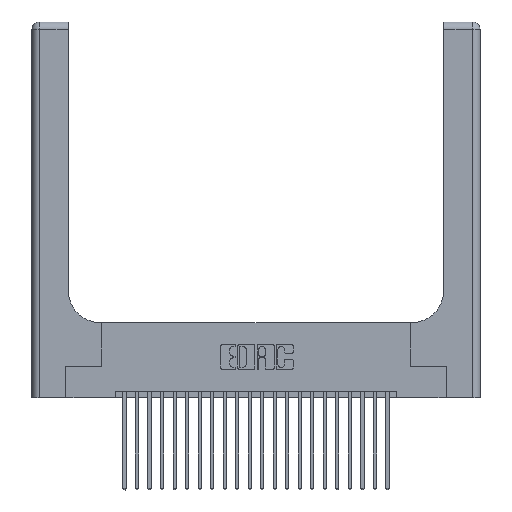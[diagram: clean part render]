
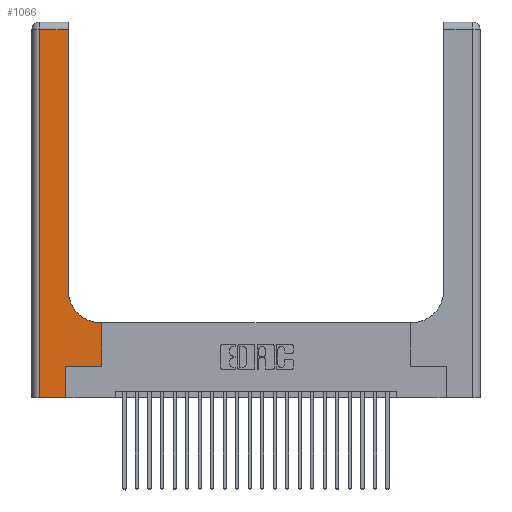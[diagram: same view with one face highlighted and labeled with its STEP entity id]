
A CAD part, top view. The second image highlights one B-rep face of the part: STEP entity #1066.
In plain terms, the highlighted planar face has unit normal (0, 0, 1).
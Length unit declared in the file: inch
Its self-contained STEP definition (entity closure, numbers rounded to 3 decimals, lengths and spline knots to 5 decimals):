
#1 = VERTEX_POINT ( 'NONE', #12243 ) ;
#51 = LINE ( 'NONE', #18129, #17416 ) ;
#165 = VERTEX_POINT ( 'NONE', #3854 ) ;
#201 = CARTESIAN_POINT ( 'NONE',  ( 0.06, 2.94, 0.37 ) ) ;
#372 = CARTESIAN_POINT ( 'NONE',  ( 0.269, 0., 0.37 ) ) ;
#1066 = ADVANCED_FACE ( 'NONE', ( #23829 ), #7288, .F. ) ;
#1139 = LINE ( 'NONE', #4367, #16083 ) ;
#1399 = ORIENTED_EDGE ( 'NONE', *, *, #13360, .T. ) ;
#2726 = DIRECTION ( 'NONE',  ( 0., 1., 0. ) ) ;
#2773 = EDGE_CURVE ( 'NONE', #1, #10433, #24336, .T. ) ;
#2787 = DIRECTION ( 'NONE',  ( 0., -1., 0. ) ) ;
#3617 = EDGE_CURVE ( 'NONE', #10433, #17808, #4555, .T. ) ;
#3854 = CARTESIAN_POINT ( 'NONE',  ( 0.2915, 2.94, 0.37 ) ) ;
#4098 = ORIENTED_EDGE ( 'NONE', *, *, #11255, .T. ) ;
#4186 = CARTESIAN_POINT ( 'NONE',  ( 0.2915, 0.6, 0.37 ) ) ;
#4367 = CARTESIAN_POINT ( 'NONE',  ( 0., 0., 0.37 ) ) ;
#4410 = CARTESIAN_POINT ( 'NONE',  ( 0.5415, 0.6, 0.37 ) ) ;
#4555 = CIRCLE ( 'NONE', #10323, 0.25 ) ;
#4596 = EDGE_CURVE ( 'NONE', #165, #16247, #18824, .T. ) ;
#5061 = ORIENTED_EDGE ( 'NONE', *, *, #21890, .T. ) ;
#5188 = CARTESIAN_POINT ( 'NONE',  ( 0.06, 0., 0.37 ) ) ;
#6261 = DIRECTION ( 'NONE',  ( 1., 0., 0. ) ) ;
#7288 = PLANE ( 'NONE',  #8512 ) ;
#7965 = CARTESIAN_POINT ( 'NONE',  ( 0., 2.94, 0.37 ) ) ;
#8123 = CARTESIAN_POINT ( 'NONE',  ( 0.269, 0.25, 0.37 ) ) ;
#8213 = EDGE_CURVE ( 'NONE', #17808, #165, #15275, .T. ) ;
#8512 = AXIS2_PLACEMENT_3D ( 'NONE', #21055, #14872, #22751 ) ;
#8567 = VECTOR ( 'NONE', #21155, 39.37008 ) ;
#8669 = DIRECTION ( 'NONE',  ( 0., 1., 0. ) ) ;
#9030 = VERTEX_POINT ( 'NONE', #372 ) ;
#10037 = VECTOR ( 'NONE', #23567, 39.37008 ) ;
#10323 = AXIS2_PLACEMENT_3D ( 'NONE', #20805, #24700, #15038 ) ;
#10433 = VERTEX_POINT ( 'NONE', #4410 ) ;
#11001 = LINE ( 'NONE', #21067, #8567 ) ;
#11255 = EDGE_CURVE ( 'NONE', #17013, #9030, #1139, .T. ) ;
#12243 = CARTESIAN_POINT ( 'NONE',  ( 0.5585, 0.6, 0.37 ) ) ;
#12869 = VERTEX_POINT ( 'NONE', #18368 ) ;
#13360 = EDGE_CURVE ( 'NONE', #16247, #17013, #19558, .T. ) ;
#14153 = DIRECTION ( 'NONE',  ( -1., 0., 0. ) ) ;
#14264 = VERTEX_POINT ( 'NONE', #19247 ) ;
#14445 = VECTOR ( 'NONE', #21695, 39.37008 ) ;
#14537 = ORIENTED_EDGE ( 'NONE', *, *, #4596, .T. ) ;
#14872 = DIRECTION ( 'NONE',  ( 0., 0., -1. ) ) ;
#15038 = DIRECTION ( 'NONE',  ( 1., 0., 0. ) ) ;
#15275 = LINE ( 'NONE', #18108, #15594 ) ;
#15594 = VECTOR ( 'NONE', #2726, 39.37008 ) ;
#16083 = VECTOR ( 'NONE', #6261, 39.37008 ) ;
#16247 = VERTEX_POINT ( 'NONE', #201 ) ;
#16311 = EDGE_CURVE ( 'NONE', #12869, #14264, #25086, .T. ) ;
#16520 = ORIENTED_EDGE ( 'NONE', *, *, #17928, .T. ) ;
#16919 = ORIENTED_EDGE ( 'NONE', *, *, #8213, .T. ) ;
#17013 = VERTEX_POINT ( 'NONE', #5188 ) ;
#17162 = CARTESIAN_POINT ( 'NONE',  ( 0.2915, 0.85, 0.37 ) ) ;
#17416 = VECTOR ( 'NONE', #8669, 39.37008 ) ;
#17808 = VERTEX_POINT ( 'NONE', #17162 ) ;
#17928 = EDGE_CURVE ( 'NONE', #14264, #1, #51, .T. ) ;
#18108 = CARTESIAN_POINT ( 'NONE',  ( 0.2915, 3., 0.37 ) ) ;
#18115 = ORIENTED_EDGE ( 'NONE', *, *, #2773, .T. ) ;
#18129 = CARTESIAN_POINT ( 'NONE',  ( 0.5585, 0.25, 0.37 ) ) ;
#18368 = CARTESIAN_POINT ( 'NONE',  ( 0.269, 0.25, 0.37 ) ) ;
#18628 = ORIENTED_EDGE ( 'NONE', *, *, #16311, .T. ) ;
#18824 = LINE ( 'NONE', #7965, #23701 ) ;
#18946 = VECTOR ( 'NONE', #2787, 39.37008 ) ;
#19247 = CARTESIAN_POINT ( 'NONE',  ( 0.5585, 0.25, 0.37 ) ) ;
#19558 = LINE ( 'NONE', #20212, #18946 ) ;
#20212 = CARTESIAN_POINT ( 'NONE',  ( 0.06, 3., 0.37 ) ) ;
#20805 = CARTESIAN_POINT ( 'NONE',  ( 0.5415, 0.85, 0.37 ) ) ;
#21055 = CARTESIAN_POINT ( 'NONE',  ( 0., 3., 0.37 ) ) ;
#21067 = CARTESIAN_POINT ( 'NONE',  ( 0.269, 0., 0.37 ) ) ;
#21155 = DIRECTION ( 'NONE',  ( 0., 1., 0. ) ) ;
#21695 = DIRECTION ( 'NONE',  ( 1., 0., 0. ) ) ;
#21890 = EDGE_CURVE ( 'NONE', #9030, #12869, #11001, .T. ) ;
#22751 = DIRECTION ( 'NONE',  ( -1., 0., 0. ) ) ;
#23358 = ORIENTED_EDGE ( 'NONE', *, *, #3617, .T. ) ;
#23567 = DIRECTION ( 'NONE',  ( -1., 0., 0. ) ) ;
#23701 = VECTOR ( 'NONE', #14153, 39.37008 ) ;
#23823 = EDGE_LOOP ( 'NONE', ( #16919, #14537, #1399, #4098, #5061, #18628, #16520, #18115, #23358 ) ) ;
#23829 = FACE_OUTER_BOUND ( 'NONE', #23823, .T. ) ;
#24336 = LINE ( 'NONE', #4186, #10037 ) ;
#24700 = DIRECTION ( 'NONE',  ( 0., 0., -1. ) ) ;
#25086 = LINE ( 'NONE', #8123, #14445 ) ;
